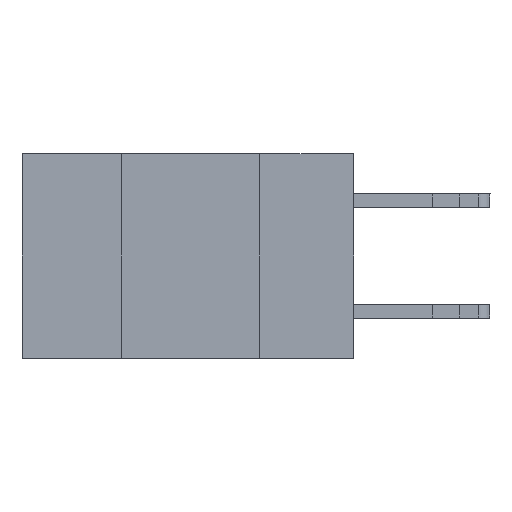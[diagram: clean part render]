
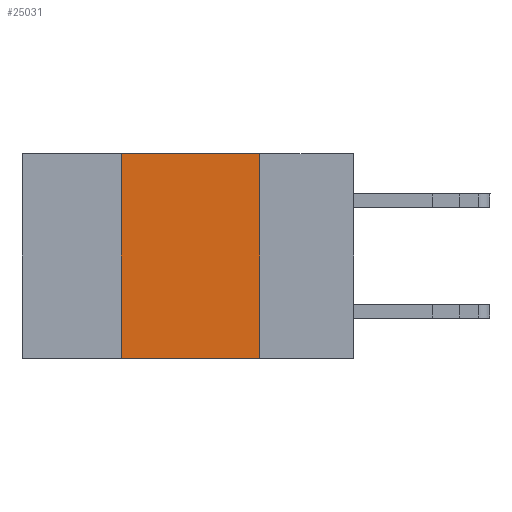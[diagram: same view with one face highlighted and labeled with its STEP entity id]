
A CAD part, left-side view. The second image highlights one B-rep face of the part: STEP entity #25031.
In plain terms, the highlighted planar face has unit normal (-1, 0, 0).
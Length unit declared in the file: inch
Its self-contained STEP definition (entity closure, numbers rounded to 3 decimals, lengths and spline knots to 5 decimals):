
#1570 = LINE ( 'NONE', #12461, #6521 ) ;
#1906 = CARTESIAN_POINT ( 'NONE',  ( 0., 0.17, 0. ) ) ;
#2162 = VERTEX_POINT ( 'NONE', #27282 ) ;
#4500 = LINE ( 'NONE', #7351, #34491 ) ;
#5969 = CARTESIAN_POINT ( 'NONE',  ( 0., 0.42, -0.37 ) ) ;
#6521 = VECTOR ( 'NONE', #23405, 39.37008 ) ;
#7351 = CARTESIAN_POINT ( 'NONE',  ( 0., 0.6, -0.37 ) ) ;
#7392 = LINE ( 'NONE', #15291, #16733 ) ;
#9093 = ORIENTED_EDGE ( 'NONE', *, *, #34936, .T. ) ;
#9674 = DIRECTION ( 'NONE',  ( 0., -1., 0. ) ) ;
#12461 = CARTESIAN_POINT ( 'NONE',  ( 0., 0.42, 0. ) ) ;
#13308 = EDGE_CURVE ( 'NONE', #31619, #2162, #1570, .T. ) ;
#13468 = DIRECTION ( 'NONE',  ( 1., 0., 0. ) ) ;
#15291 = CARTESIAN_POINT ( 'NONE',  ( 0., 0.6, 0. ) ) ;
#16316 = ORIENTED_EDGE ( 'NONE', *, *, #13308, .F. ) ;
#16733 = VECTOR ( 'NONE', #34483, 39.37008 ) ;
#19050 = FACE_OUTER_BOUND ( 'NONE', #34174, .T. ) ;
#20230 = CARTESIAN_POINT ( 'NONE',  ( 0., 0.17, -0.37 ) ) ;
#20710 = DIRECTION ( 'NONE',  ( 0., 0., -1. ) ) ;
#21081 = VERTEX_POINT ( 'NONE', #1906 ) ;
#21641 = EDGE_CURVE ( 'NONE', #21081, #35201, #25418, .T. ) ;
#23405 = DIRECTION ( 'NONE',  ( 0., 0., 1. ) ) ;
#24046 = VECTOR ( 'NONE', #25592, 39.37008 ) ;
#24906 = CARTESIAN_POINT ( 'NONE',  ( 0., 0.17, 0. ) ) ;
#25031 = ADVANCED_FACE ( 'NONE', ( #19050 ), #28932, .F. ) ;
#25418 = LINE ( 'NONE', #24906, #24046 ) ;
#25592 = DIRECTION ( 'NONE',  ( 0., 0., -1. ) ) ;
#27223 = AXIS2_PLACEMENT_3D ( 'NONE', #34334, #13468, #20710 ) ;
#27282 = CARTESIAN_POINT ( 'NONE',  ( 0., 0.42, 0. ) ) ;
#28932 = PLANE ( 'NONE',  #27223 ) ;
#30886 = ORIENTED_EDGE ( 'NONE', *, *, #21641, .F. ) ;
#31619 = VERTEX_POINT ( 'NONE', #5969 ) ;
#34174 = EDGE_LOOP ( 'NONE', ( #30886, #34842, #16316, #9093 ) ) ;
#34334 = CARTESIAN_POINT ( 'NONE',  ( 0., 0.6, 0. ) ) ;
#34454 = EDGE_CURVE ( 'NONE', #2162, #21081, #7392, .T. ) ;
#34483 = DIRECTION ( 'NONE',  ( 0., -1., 0. ) ) ;
#34491 = VECTOR ( 'NONE', #9674, 39.37008 ) ;
#34842 = ORIENTED_EDGE ( 'NONE', *, *, #34454, .F. ) ;
#34936 = EDGE_CURVE ( 'NONE', #31619, #35201, #4500, .T. ) ;
#35201 = VERTEX_POINT ( 'NONE', #20230 ) ;
